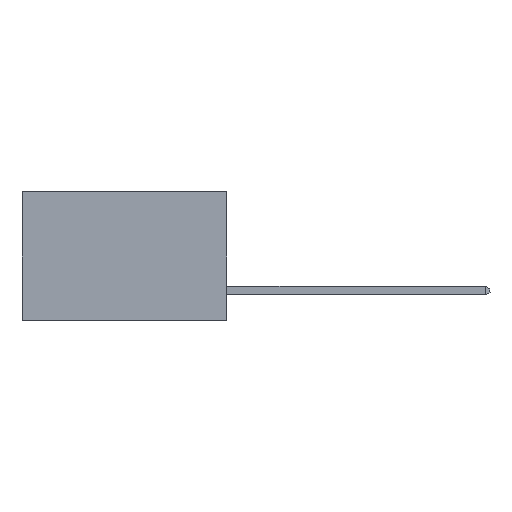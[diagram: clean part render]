
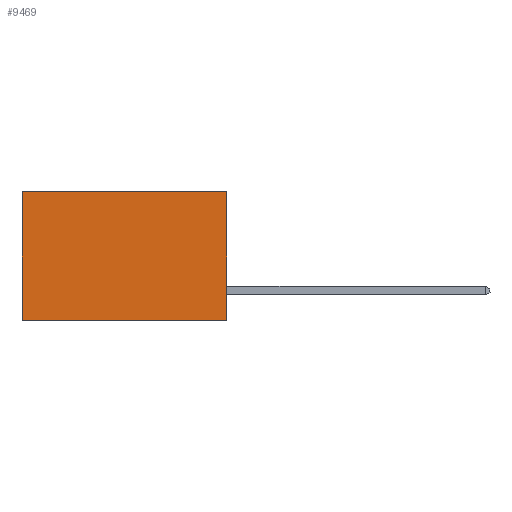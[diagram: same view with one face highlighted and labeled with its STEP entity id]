
A CAD part, left-side view. The second image highlights one B-rep face of the part: STEP entity #9469.
In plain terms, the highlighted planar face has unit normal (-1, 0, 0).
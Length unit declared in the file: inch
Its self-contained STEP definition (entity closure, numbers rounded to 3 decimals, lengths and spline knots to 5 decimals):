
#1395 = PLANE ( 'NONE',  #12226 ) ;
#1682 = CARTESIAN_POINT ( 'NONE',  ( 0.277, 0., 0. ) ) ;
#2255 = LINE ( 'NONE', #8140, #13191 ) ;
#2489 = CARTESIAN_POINT ( 'NONE',  ( 0.277, 0., -0.37 ) ) ;
#2520 = DIRECTION ( 'NONE',  ( 1., 0., 0. ) ) ;
#3069 = CARTESIAN_POINT ( 'NONE',  ( 0.277, 0., -0.37 ) ) ;
#4243 = CARTESIAN_POINT ( 'NONE',  ( 0.277, 0., -0.37 ) ) ;
#4530 = CARTESIAN_POINT ( 'NONE',  ( 0.277, 0.59, -0.37 ) ) ;
#5043 = DIRECTION ( 'NONE',  ( 0., 1., 0. ) ) ;
#5401 = LINE ( 'NONE', #2489, #7963 ) ;
#5836 = VECTOR ( 'NONE', #13593, 39.37008 ) ;
#5869 = CARTESIAN_POINT ( 'NONE',  ( 0.277, 0., 0. ) ) ;
#5919 = EDGE_CURVE ( 'NONE', #8563, #7569, #2255, .T. ) ;
#6772 = DIRECTION ( 'NONE',  ( 0., 0., -1. ) ) ;
#7171 = FACE_OUTER_BOUND ( 'NONE', #11395, .T. ) ;
#7569 = VERTEX_POINT ( 'NONE', #4530 ) ;
#7963 = VECTOR ( 'NONE', #8055, 39.37008 ) ;
#8055 = DIRECTION ( 'NONE',  ( 0., 1., 0. ) ) ;
#8140 = CARTESIAN_POINT ( 'NONE',  ( 0.277, 0.59, -0.37 ) ) ;
#8563 = VERTEX_POINT ( 'NONE', #10489 ) ;
#9108 = CARTESIAN_POINT ( 'NONE',  ( 0.277, 0., -0.37 ) ) ;
#9153 = EDGE_CURVE ( 'NONE', #11819, #12757, #13701, .T. ) ;
#9290 = ORIENTED_EDGE ( 'NONE', *, *, #5919, .T. ) ;
#9469 = ADVANCED_FACE ( 'NONE', ( #7171 ), #1395, .F. ) ;
#9764 = ORIENTED_EDGE ( 'NONE', *, *, #11214, .F. ) ;
#10167 = DIRECTION ( 'NONE',  ( 0., 0., -1. ) ) ;
#10489 = CARTESIAN_POINT ( 'NONE',  ( 0.277, 0.59, 0. ) ) ;
#10756 = VECTOR ( 'NONE', #5043, 39.37008 ) ;
#10812 = EDGE_CURVE ( 'NONE', #11819, #8563, #11067, .T. ) ;
#11067 = LINE ( 'NONE', #1682, #10756 ) ;
#11110 = ORIENTED_EDGE ( 'NONE', *, *, #9153, .F. ) ;
#11214 = EDGE_CURVE ( 'NONE', #12757, #7569, #5401, .T. ) ;
#11360 = ORIENTED_EDGE ( 'NONE', *, *, #10812, .T. ) ;
#11395 = EDGE_LOOP ( 'NONE', ( #9290, #9764, #11110, #11360 ) ) ;
#11819 = VERTEX_POINT ( 'NONE', #5869 ) ;
#12226 = AXIS2_PLACEMENT_3D ( 'NONE', #9108, #2520, #10167 ) ;
#12757 = VERTEX_POINT ( 'NONE', #4243 ) ;
#13191 = VECTOR ( 'NONE', #6772, 39.37008 ) ;
#13593 = DIRECTION ( 'NONE',  ( 0., 0., -1. ) ) ;
#13701 = LINE ( 'NONE', #3069, #5836 ) ;
